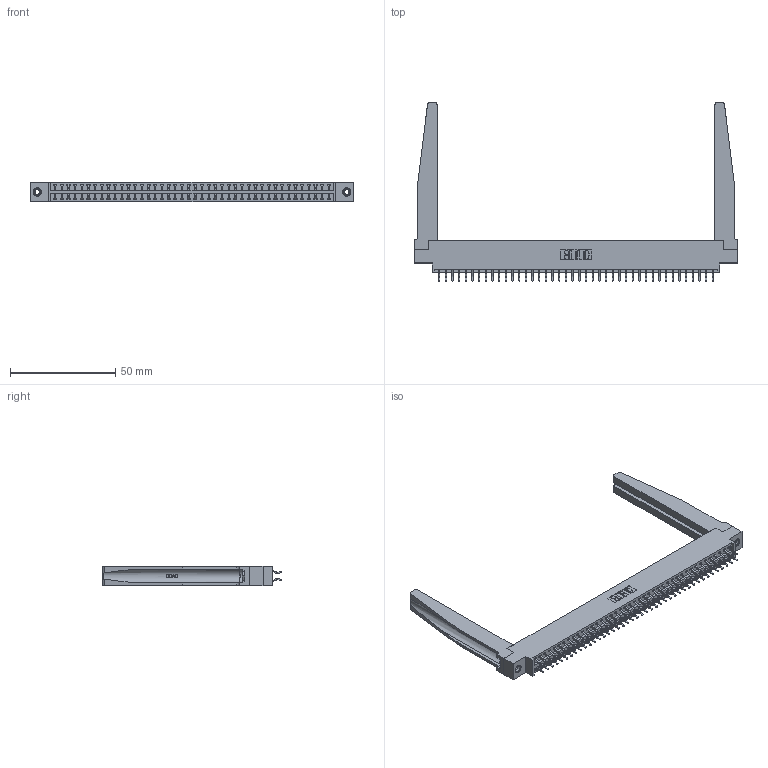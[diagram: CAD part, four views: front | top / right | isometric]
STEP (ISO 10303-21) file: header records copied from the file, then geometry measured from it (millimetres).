
FILE_DESCRIPTION (( 'STEP AP203' ), '1' );
FILE_NAME ('346-084-556-878.STEP', '2022-05-25T20:47:02', ( '' ), ( '' ), 'SwSTEP 2.0', 'SolidWorks 2020', '' );
FILE_SCHEMA (( 'CONFIG_CONTROL_DESIGN' ));
Length unit declared in the file: inch
Products named in the file (5): 345-250-001_345-250-001-102; 346 Part_0.170 Offset - 0.156 Dia-TH; 346-220-078_345-220-078; 346-084-556-878; 345-292-001_556 Tail
Assembly tree (89 placements, depth 2):
  346-084-556-878
    346 Part_0.170 Offset - 0.156 Dia-TH
    345-292-001_556 Tail  x84
    346-220-078_345-220-078  x2
    345-250-001_345-250-001-102  x2
Bounding box: 153.92 x 84.84 x 9.4 mm (x, y, z)
Volume: 21742.3 mm3; surface area: 27063.2 mm2
Topology: 89 solids, 89 shells, 5246 faces, 15517 edges, 10222 vertices
Faces by surface type: plane 3512, cylinder 1682, bspline 36, cone 12, torus 4
Entity records: 32926 total; most frequent: CARTESIAN_POINT 6385, ORIENTED_EDGE 5194, DIRECTION 4651, EDGE_CURVE 2597, LINE 2195, VECTOR 2195, VERTEX_POINT 1724, AXIS2_PLACEMENT_3D 1228
